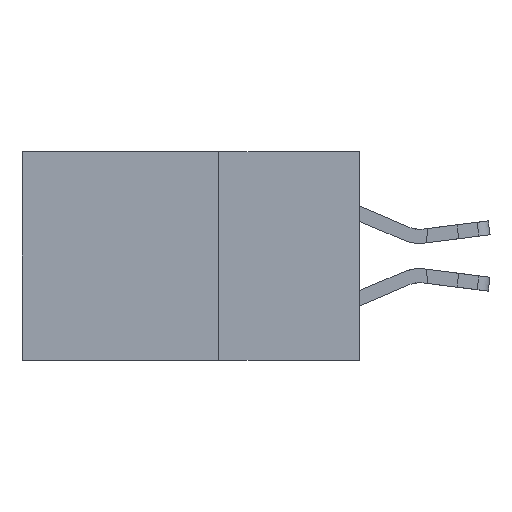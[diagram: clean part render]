
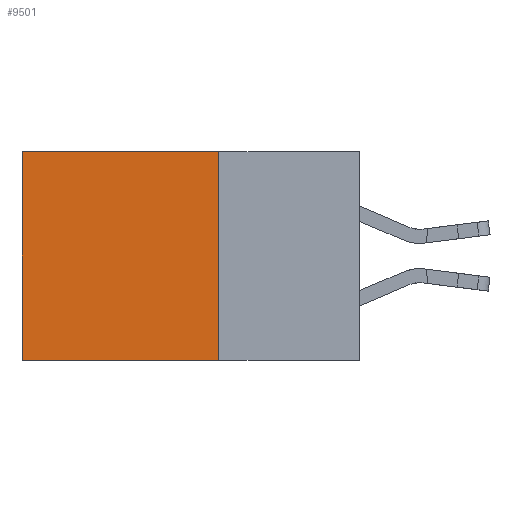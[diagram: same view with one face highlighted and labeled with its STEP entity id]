
A CAD part, left-side view. The second image highlights one B-rep face of the part: STEP entity #9501.
In plain terms, the highlighted planar face has unit normal (-1, 0, 0).
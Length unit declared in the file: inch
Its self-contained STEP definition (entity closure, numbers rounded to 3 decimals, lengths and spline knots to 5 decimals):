
#111 = EDGE_LOOP ( 'NONE', ( #5192, #5931, #6442, #5092 ) ) ;
#1068 = VERTEX_POINT ( 'NONE', #12938 ) ;
#1358 = PLANE ( 'NONE',  #12673 ) ;
#1411 = VECTOR ( 'NONE', #7322, 39.37008 ) ;
#1441 = EDGE_CURVE ( 'NONE', #17168, #3806, #1814, .T. ) ;
#1630 = VECTOR ( 'NONE', #4821, 39.37008 ) ;
#1814 = LINE ( 'NONE', #7595, #1411 ) ;
#2011 = EDGE_CURVE ( 'NONE', #17168, #9742, #2441, .T. ) ;
#2441 = LINE ( 'NONE', #9211, #4813 ) ;
#2917 = DIRECTION ( 'NONE',  ( 1., 0., 0. ) ) ;
#3461 = LINE ( 'NONE', #17483, #1630 ) ;
#3510 = CARTESIAN_POINT ( 'NONE',  ( 0.2875, 0.6, 0. ) ) ;
#3806 = VERTEX_POINT ( 'NONE', #15976 ) ;
#4686 = LINE ( 'NONE', #3510, #12526 ) ;
#4813 = VECTOR ( 'NONE', #17570, 39.37008 ) ;
#4821 = DIRECTION ( 'NONE',  ( 0., 1., 0. ) ) ;
#5092 = ORIENTED_EDGE ( 'NONE', *, *, #2011, .T. ) ;
#5192 = ORIENTED_EDGE ( 'NONE', *, *, #15650, .T. ) ;
#5293 = CARTESIAN_POINT ( 'NONE',  ( 0.2875, 0.6, 0. ) ) ;
#5841 = CARTESIAN_POINT ( 'NONE',  ( 0.2875, 0.25, 0. ) ) ;
#5931 = ORIENTED_EDGE ( 'NONE', *, *, #13343, .F. ) ;
#6442 = ORIENTED_EDGE ( 'NONE', *, *, #1441, .F. ) ;
#7037 = DIRECTION ( 'NONE',  ( 0., 0., -1. ) ) ;
#7322 = DIRECTION ( 'NONE',  ( 0., 0., -1. ) ) ;
#7595 = CARTESIAN_POINT ( 'NONE',  ( 0.2875, 0.25, 0. ) ) ;
#7716 = DIRECTION ( 'NONE',  ( 0., 0., -1. ) ) ;
#9211 = CARTESIAN_POINT ( 'NONE',  ( 0.2875, 0.25, 0. ) ) ;
#9501 = ADVANCED_FACE ( 'NONE', ( #12894 ), #1358, .F. ) ;
#9742 = VERTEX_POINT ( 'NONE', #5293 ) ;
#12526 = VECTOR ( 'NONE', #7716, 39.37008 ) ;
#12673 = AXIS2_PLACEMENT_3D ( 'NONE', #13987, #2917, #7037 ) ;
#12894 = FACE_OUTER_BOUND ( 'NONE', #111, .T. ) ;
#12938 = CARTESIAN_POINT ( 'NONE',  ( 0.2875, 0.6, -0.37 ) ) ;
#13343 = EDGE_CURVE ( 'NONE', #3806, #1068, #3461, .T. ) ;
#13987 = CARTESIAN_POINT ( 'NONE',  ( 0.2875, 0.25, 0. ) ) ;
#15650 = EDGE_CURVE ( 'NONE', #9742, #1068, #4686, .T. ) ;
#15976 = CARTESIAN_POINT ( 'NONE',  ( 0.2875, 0.25, -0.37 ) ) ;
#17168 = VERTEX_POINT ( 'NONE', #5841 ) ;
#17483 = CARTESIAN_POINT ( 'NONE',  ( 0.2875, 0.25, -0.37 ) ) ;
#17570 = DIRECTION ( 'NONE',  ( 0., 1., 0. ) ) ;
